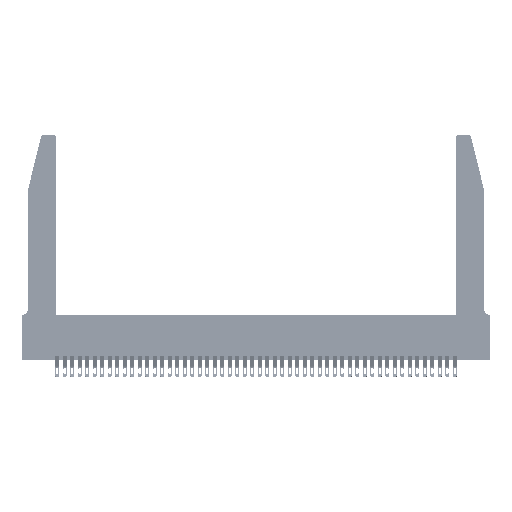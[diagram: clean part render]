
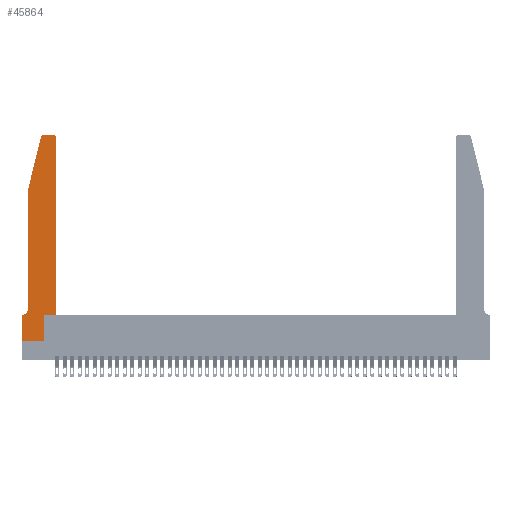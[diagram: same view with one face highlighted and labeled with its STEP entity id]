
A CAD part, top view. The second image highlights one B-rep face of the part: STEP entity #45864.
In plain terms, the highlighted planar face has unit normal (0, 0, 1).
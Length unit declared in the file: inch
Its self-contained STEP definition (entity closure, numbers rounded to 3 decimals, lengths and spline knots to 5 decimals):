
#1013 = CARTESIAN_POINT ( 'NONE',  ( 0.4505, 0.35, 0.37 ) ) ;
#1312 = VERTEX_POINT ( 'NONE', #3255 ) ;
#1826 = CARTESIAN_POINT ( 'NONE',  ( 0.4205, 2.72, 0.37 ) ) ;
#1898 = ORIENTED_EDGE ( 'NONE', *, *, #9571, .T. ) ;
#2580 = CARTESIAN_POINT ( 'NONE',  ( 0.0055, 0.42, 0.37 ) ) ;
#3255 = CARTESIAN_POINT ( 'NONE',  ( 0.4205, 2.75, 0.37 ) ) ;
#4268 = LINE ( 'NONE', #1013, #31536 ) ;
#4478 = EDGE_CURVE ( 'NONE', #1312, #29747, #34777, .T. ) ;
#4543 = EDGE_CURVE ( 'NONE', #21193, #4901, #4268, .T. ) ;
#4901 = VERTEX_POINT ( 'NONE', #25314 ) ;
#5330 = ORIENTED_EDGE ( 'NONE', *, *, #36877, .T. ) ;
#5503 = DIRECTION ( 'NONE',  ( 1., 0., 0. ) ) ;
#5888 = ORIENTED_EDGE ( 'NONE', *, *, #10871, .T. ) ;
#6232 = DIRECTION ( 'NONE',  ( -1., 0., 0. ) ) ;
#6334 = DIRECTION ( 'NONE',  ( 0., 0., 1. ) ) ;
#6844 = DIRECTION ( 'NONE',  ( 1., 0., 0. ) ) ;
#7445 = CARTESIAN_POINT ( 'NONE',  ( 0.4505, 2.72, 0.37 ) ) ;
#7834 = AXIS2_PLACEMENT_3D ( 'NONE', #2580, #27579, #6232 ) ;
#7839 = DIRECTION ( 'NONE',  ( -1., 0., 0. ) ) ;
#8198 = EDGE_CURVE ( 'NONE', #24572, #1312, #33972, .T. ) ;
#9571 = EDGE_CURVE ( 'NONE', #21057, #40051, #23650, .T. ) ;
#10094 = LINE ( 'NONE', #39009, #26784 ) ;
#10871 = EDGE_CURVE ( 'NONE', #4901, #24572, #10094, .T. ) ;
#11120 = VERTEX_POINT ( 'NONE', #15981 ) ;
#11645 = DIRECTION ( 'NONE',  ( -1., 0., 0. ) ) ;
#12105 = EDGE_LOOP ( 'NONE', ( #19326, #19869, #35857, #32593, #40178, #5330, #21092, #1898, #24353, #18251, #5888, #17722 ) ) ;
#12335 = FACE_OUTER_BOUND ( 'NONE', #12105, .T. ) ;
#12745 = DIRECTION ( 'NONE',  ( 0., -1., 0. ) ) ;
#14106 = CIRCLE ( 'NONE', #33093, 0.03 ) ;
#14157 = VECTOR ( 'NONE', #6844, 39.37008 ) ;
#15981 = CARTESIAN_POINT ( 'NONE',  ( 0.0755, 0.42, 0.37 ) ) ;
#16292 = VECTOR ( 'NONE', #43047, 39.37008 ) ;
#16460 = CARTESIAN_POINT ( 'NONE',  ( 0., 0.35, 0.37 ) ) ;
#16692 = DIRECTION ( 'NONE',  ( 0., 1., 0. ) ) ;
#17440 = CARTESIAN_POINT ( 'NONE',  ( 0., 0.35, 0.37 ) ) ;
#17703 = CARTESIAN_POINT ( 'NONE',  ( 0.0755, 2., 0.37 ) ) ;
#17722 = ORIENTED_EDGE ( 'NONE', *, *, #8198, .T. ) ;
#18251 = ORIENTED_EDGE ( 'NONE', *, *, #4543, .T. ) ;
#18726 = CARTESIAN_POINT ( 'NONE',  ( 0.0755, 0.35, 0.37 ) ) ;
#19302 = VERTEX_POINT ( 'NONE', #42696 ) ;
#19326 = ORIENTED_EDGE ( 'NONE', *, *, #4478, .T. ) ;
#19869 = ORIENTED_EDGE ( 'NONE', *, *, #45114, .T. ) ;
#20247 = LINE ( 'NONE', #44384, #28463 ) ;
#21050 = DIRECTION ( 'NONE',  ( 0., 0., 1. ) ) ;
#21057 = VERTEX_POINT ( 'NONE', #31744 ) ;
#21092 = ORIENTED_EDGE ( 'NONE', *, *, #45649, .T. ) ;
#21193 = VERTEX_POINT ( 'NONE', #42855 ) ;
#21660 = DIRECTION ( 'NONE',  ( 0., 1., 0. ) ) ;
#21860 = LINE ( 'NONE', #34180, #22938 ) ;
#22562 = DIRECTION ( 'NONE',  ( 1., 0., 0. ) ) ;
#22719 = VERTEX_POINT ( 'NONE', #41184 ) ;
#22938 = VECTOR ( 'NONE', #16692, 39.37008 ) ;
#23528 = VECTOR ( 'NONE', #11645, 39.37008 ) ;
#23650 = LINE ( 'NONE', #42177, #14157 ) ;
#24353 = ORIENTED_EDGE ( 'NONE', *, *, #37148, .T. ) ;
#24572 = VERTEX_POINT ( 'NONE', #7445 ) ;
#25157 = VECTOR ( 'NONE', #12745, 39.37008 ) ;
#25314 = CARTESIAN_POINT ( 'NONE',  ( 0.4505, 0.35, 0.37 ) ) ;
#25529 = VECTOR ( 'NONE', #7839, 39.37008 ) ;
#26141 = AXIS2_PLACEMENT_3D ( 'NONE', #1826, #26865, #5503 ) ;
#26784 = VECTOR ( 'NONE', #21660, 39.37008 ) ;
#26865 = DIRECTION ( 'NONE',  ( 0., 0., 1. ) ) ;
#27027 = DIRECTION ( 'NONE',  ( 0., -1., 0. ) ) ;
#27579 = DIRECTION ( 'NONE',  ( 0., 0., -1. ) ) ;
#27679 = CARTESIAN_POINT ( 'NONE',  ( 0.284, 2.72, 0.37 ) ) ;
#28463 = VECTOR ( 'NONE', #27027, 39.37008 ) ;
#29747 = VERTEX_POINT ( 'NONE', #40270 ) ;
#31197 = DIRECTION ( 'NONE',  ( 1., 0., 0. ) ) ;
#31536 = VECTOR ( 'NONE', #22562, 39.37008 ) ;
#31744 = CARTESIAN_POINT ( 'NONE',  ( 0., 0., 0.37 ) ) ;
#32593 = ORIENTED_EDGE ( 'NONE', *, *, #37082, .T. ) ;
#32797 = LINE ( 'NONE', #18726, #23528 ) ;
#33093 = AXIS2_PLACEMENT_3D ( 'NONE', #27679, #6334, #31197 ) ;
#33881 = CARTESIAN_POINT ( 'NONE',  ( 0.0755, 2., 0.37 ) ) ;
#33972 = CIRCLE ( 'NONE', #26141, 0.03 ) ;
#34180 = CARTESIAN_POINT ( 'NONE',  ( 0.2865, 0.35, 0.37 ) ) ;
#34404 = LINE ( 'NONE', #33881, #25157 ) ;
#34574 = CARTESIAN_POINT ( 'NONE',  ( 0.2865, 0., 0.37 ) ) ;
#34777 = LINE ( 'NONE', #43011, #25529 ) ;
#35857 = ORIENTED_EDGE ( 'NONE', *, *, #36809, .T. ) ;
#36809 = EDGE_CURVE ( 'NONE', #19302, #37961, #44243, .T. ) ;
#36877 = EDGE_CURVE ( 'NONE', #22719, #41988, #32797, .T. ) ;
#37082 = EDGE_CURVE ( 'NONE', #37961, #11120, #34404, .T. ) ;
#37148 = EDGE_CURVE ( 'NONE', #40051, #21193, #21860, .T. ) ;
#37742 = CIRCLE ( 'NONE', #7834, 0.07 ) ;
#37961 = VERTEX_POINT ( 'NONE', #17703 ) ;
#38418 = PLANE ( 'NONE',  #40687 ) ;
#39009 = CARTESIAN_POINT ( 'NONE',  ( 0.4505, 0.35, 0.37 ) ) ;
#39508 = CARTESIAN_POINT ( 'NONE',  ( 0.0755, 2., 0.37 ) ) ;
#40051 = VERTEX_POINT ( 'NONE', #34574 ) ;
#40178 = ORIENTED_EDGE ( 'NONE', *, *, #44516, .T. ) ;
#40270 = CARTESIAN_POINT ( 'NONE',  ( 0.284, 2.75, 0.37 ) ) ;
#40687 = AXIS2_PLACEMENT_3D ( 'NONE', #17440, #21050, #45435 ) ;
#41184 = CARTESIAN_POINT ( 'NONE',  ( 0.0055, 0.35, 0.37 ) ) ;
#41988 = VERTEX_POINT ( 'NONE', #16460 ) ;
#42177 = CARTESIAN_POINT ( 'NONE',  ( 0., 0., 0.37 ) ) ;
#42696 = CARTESIAN_POINT ( 'NONE',  ( 0.25487, 2.72718, 0.37 ) ) ;
#42855 = CARTESIAN_POINT ( 'NONE',  ( 0.2865, 0.35, 0.37 ) ) ;
#43011 = CARTESIAN_POINT ( 'NONE',  ( 0.2605, 2.75, 0.37 ) ) ;
#43047 = DIRECTION ( 'NONE',  ( -0.239, -0.971, 0. ) ) ;
#44243 = LINE ( 'NONE', #39508, #16292 ) ;
#44384 = CARTESIAN_POINT ( 'NONE',  ( 0., 0., 0.37 ) ) ;
#44516 = EDGE_CURVE ( 'NONE', #11120, #22719, #37742, .T. ) ;
#45114 = EDGE_CURVE ( 'NONE', #29747, #19302, #14106, .T. ) ;
#45435 = DIRECTION ( 'NONE',  ( 1., 0., 0. ) ) ;
#45649 = EDGE_CURVE ( 'NONE', #41988, #21057, #20247, .T. ) ;
#45864 = ADVANCED_FACE ( 'NONE', ( #12335 ), #38418, .T. ) ;
